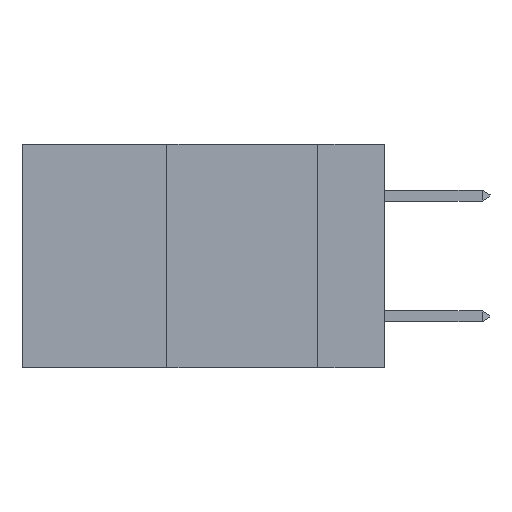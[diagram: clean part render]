
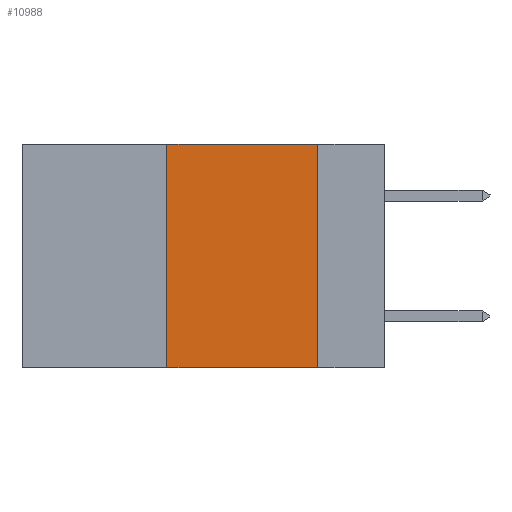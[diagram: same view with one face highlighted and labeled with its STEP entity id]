
A CAD part, left-side view. The second image highlights one B-rep face of the part: STEP entity #10988.
In plain terms, the highlighted planar face has unit normal (-1, 0, 0).
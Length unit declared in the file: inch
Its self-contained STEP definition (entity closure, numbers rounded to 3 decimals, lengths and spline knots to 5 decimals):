
#573 = DIRECTION ( 'NONE',  ( 0., -1., 0. ) ) ;
#1164 = ORIENTED_EDGE ( 'NONE', *, *, #28416, .T. ) ;
#3387 = VECTOR ( 'NONE', #10004, 39.37008 ) ;
#3443 = VERTEX_POINT ( 'NONE', #20548 ) ;
#5235 = AXIS2_PLACEMENT_3D ( 'NONE', #28304, #25281, #23096 ) ;
#5633 = VERTEX_POINT ( 'NONE', #9116 ) ;
#6084 = CARTESIAN_POINT ( 'NONE',  ( 0., 0.36, 0. ) ) ;
#6806 = EDGE_CURVE ( 'NONE', #31859, #17429, #31584, .T. ) ;
#7004 = VECTOR ( 'NONE', #29154, 39.37008 ) ;
#9116 = CARTESIAN_POINT ( 'NONE',  ( 0., 0.11, 0. ) ) ;
#10004 = DIRECTION ( 'NONE',  ( 0., 0., 1. ) ) ;
#10560 = VECTOR ( 'NONE', #23909, 39.37008 ) ;
#10988 = ADVANCED_FACE ( 'NONE', ( #33847 ), #35787, .F. ) ;
#11124 = VECTOR ( 'NONE', #573, 39.37008 ) ;
#13542 = LINE ( 'NONE', #26092, #7004 ) ;
#15575 = CARTESIAN_POINT ( 'NONE',  ( 0., 0.11, 0. ) ) ;
#15984 = EDGE_CURVE ( 'NONE', #17429, #5633, #24153, .T. ) ;
#16769 = ORIENTED_EDGE ( 'NONE', *, *, #6806, .F. ) ;
#17429 = VERTEX_POINT ( 'NONE', #6084 ) ;
#20548 = CARTESIAN_POINT ( 'NONE',  ( 0., 0.11, -0.37 ) ) ;
#20551 = LINE ( 'NONE', #15575, #10560 ) ;
#22888 = CARTESIAN_POINT ( 'NONE',  ( 0., 0.36, -0.37 ) ) ;
#23096 = DIRECTION ( 'NONE',  ( 0., 0., -1. ) ) ;
#23451 = CARTESIAN_POINT ( 'NONE',  ( 0., 0.36, 0. ) ) ;
#23909 = DIRECTION ( 'NONE',  ( 0., 0., -1. ) ) ;
#24153 = LINE ( 'NONE', #25674, #11124 ) ;
#25281 = DIRECTION ( 'NONE',  ( 1., 0., 0. ) ) ;
#25674 = CARTESIAN_POINT ( 'NONE',  ( 0., 0.6, 0. ) ) ;
#26092 = CARTESIAN_POINT ( 'NONE',  ( 0., 0.6, -0.37 ) ) ;
#28304 = CARTESIAN_POINT ( 'NONE',  ( 0., 0.6, 0. ) ) ;
#28416 = EDGE_CURVE ( 'NONE', #31859, #3443, #13542, .T. ) ;
#28727 = ORIENTED_EDGE ( 'NONE', *, *, #35581, .F. ) ;
#29154 = DIRECTION ( 'NONE',  ( 0., -1., 0. ) ) ;
#30513 = EDGE_LOOP ( 'NONE', ( #28727, #31974, #16769, #1164 ) ) ;
#31584 = LINE ( 'NONE', #23451, #3387 ) ;
#31859 = VERTEX_POINT ( 'NONE', #22888 ) ;
#31974 = ORIENTED_EDGE ( 'NONE', *, *, #15984, .F. ) ;
#33847 = FACE_OUTER_BOUND ( 'NONE', #30513, .T. ) ;
#35581 = EDGE_CURVE ( 'NONE', #5633, #3443, #20551, .T. ) ;
#35787 = PLANE ( 'NONE',  #5235 ) ;
